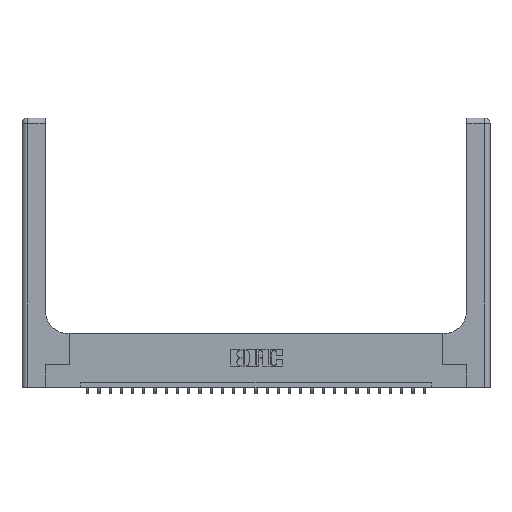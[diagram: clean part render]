
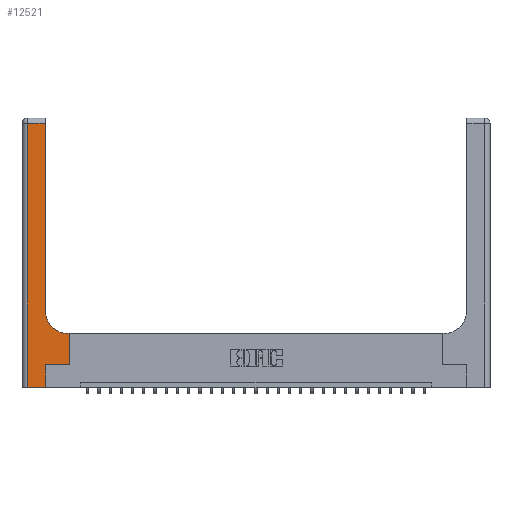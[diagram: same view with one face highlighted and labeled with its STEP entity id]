
A CAD part, top view. The second image highlights one B-rep face of the part: STEP entity #12521.
In plain terms, the highlighted planar face has unit normal (0, 0, 1).
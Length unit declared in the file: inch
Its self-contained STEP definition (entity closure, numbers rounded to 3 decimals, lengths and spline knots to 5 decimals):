
#50 = DIRECTION ( 'NONE',  ( 1., 0., 0. ) ) ;
#111 = CARTESIAN_POINT ( 'NONE',  ( 0.265, 0., 0.37 ) ) ;
#427 = VERTEX_POINT ( 'NONE', #14465 ) ;
#532 = ORIENTED_EDGE ( 'NONE', *, *, #23158, .T. ) ;
#588 = CARTESIAN_POINT ( 'NONE',  ( 0.528, 0.6, 0.37 ) ) ;
#691 = VECTOR ( 'NONE', #22587, 39.37008 ) ;
#862 = ORIENTED_EDGE ( 'NONE', *, *, #18617, .T. ) ;
#1159 = CARTESIAN_POINT ( 'NONE',  ( 0.528, 0.25, 0.37 ) ) ;
#1167 = ORIENTED_EDGE ( 'NONE', *, *, #24112, .T. ) ;
#1760 = EDGE_CURVE ( 'NONE', #3355, #6102, #11628, .T. ) ;
#1954 = ORIENTED_EDGE ( 'NONE', *, *, #11240, .T. ) ;
#2150 = DIRECTION ( 'NONE',  ( 0., 1., 0. ) ) ;
#2804 = AXIS2_PLACEMENT_3D ( 'NONE', #19322, #7292, #21332 ) ;
#3355 = VERTEX_POINT ( 'NONE', #23762 ) ;
#4939 = ORIENTED_EDGE ( 'NONE', *, *, #1760, .T. ) ;
#4972 = CARTESIAN_POINT ( 'NONE',  ( 0.06, 2.94, 0.37 ) ) ;
#5328 = EDGE_CURVE ( 'NONE', #8475, #16915, #11083, .T. ) ;
#5353 = DIRECTION ( 'NONE',  ( 0., 1., 0. ) ) ;
#5965 = CIRCLE ( 'NONE', #2804, 0.25 ) ;
#6033 = FACE_OUTER_BOUND ( 'NONE', #18383, .T. ) ;
#6042 = PLANE ( 'NONE',  #8187 ) ;
#6102 = VERTEX_POINT ( 'NONE', #4972 ) ;
#7292 = DIRECTION ( 'NONE',  ( 0., 0., -1. ) ) ;
#7917 = LINE ( 'NONE', #20095, #23245 ) ;
#8114 = DIRECTION ( 'NONE',  ( 0., 0., -1. ) ) ;
#8163 = LINE ( 'NONE', #12477, #17531 ) ;
#8187 = AXIS2_PLACEMENT_3D ( 'NONE', #24016, #8114, #22113 ) ;
#8475 = VERTEX_POINT ( 'NONE', #588 ) ;
#8661 = LINE ( 'NONE', #23739, #18674 ) ;
#9267 = LINE ( 'NONE', #111, #18015 ) ;
#9355 = EDGE_CURVE ( 'NONE', #427, #17977, #8661, .T. ) ;
#9898 = EDGE_CURVE ( 'NONE', #12443, #427, #9267, .T. ) ;
#10510 = DIRECTION ( 'NONE',  ( -1., 0., 0. ) ) ;
#10623 = CARTESIAN_POINT ( 'NONE',  ( 0.06, 3., 0.37 ) ) ;
#11083 = LINE ( 'NONE', #24469, #21079 ) ;
#11094 = VERTEX_POINT ( 'NONE', #13702 ) ;
#11240 = EDGE_CURVE ( 'NONE', #11094, #12443, #7917, .T. ) ;
#11435 = LINE ( 'NONE', #10623, #691 ) ;
#11628 = LINE ( 'NONE', #15218, #15021 ) ;
#11678 = ORIENTED_EDGE ( 'NONE', *, *, #9898, .T. ) ;
#12443 = VERTEX_POINT ( 'NONE', #23836 ) ;
#12477 = CARTESIAN_POINT ( 'NONE',  ( 0.528, 0.25, 0.37 ) ) ;
#12521 = ADVANCED_FACE ( 'NONE', ( #6033 ), #6042, .F. ) ;
#13414 = VECTOR ( 'NONE', #5353, 39.37008 ) ;
#13702 = CARTESIAN_POINT ( 'NONE',  ( 0.06, 0., 0.37 ) ) ;
#13934 = ORIENTED_EDGE ( 'NONE', *, *, #9355, .T. ) ;
#14465 = CARTESIAN_POINT ( 'NONE',  ( 0.265, 0.25, 0.37 ) ) ;
#15021 = VECTOR ( 'NONE', #21262, 39.37008 ) ;
#15218 = CARTESIAN_POINT ( 'NONE',  ( 0., 2.94, 0.37 ) ) ;
#15515 = CARTESIAN_POINT ( 'NONE',  ( 0.26, 0.85, 0.37 ) ) ;
#16285 = ORIENTED_EDGE ( 'NONE', *, *, #5328, .T. ) ;
#16915 = VERTEX_POINT ( 'NONE', #17501 ) ;
#17066 = ORIENTED_EDGE ( 'NONE', *, *, #21634, .T. ) ;
#17501 = CARTESIAN_POINT ( 'NONE',  ( 0.51, 0.6, 0.37 ) ) ;
#17531 = VECTOR ( 'NONE', #24419, 39.37008 ) ;
#17977 = VERTEX_POINT ( 'NONE', #1159 ) ;
#18015 = VECTOR ( 'NONE', #2150, 39.37008 ) ;
#18383 = EDGE_LOOP ( 'NONE', ( #862, #4939, #17066, #1954, #11678, #13934, #1167, #16285, #532 ) ) ;
#18617 = EDGE_CURVE ( 'NONE', #25526, #3355, #24050, .T. ) ;
#18674 = VECTOR ( 'NONE', #25737, 39.37008 ) ;
#19322 = CARTESIAN_POINT ( 'NONE',  ( 0.51, 0.85, 0.37 ) ) ;
#20095 = CARTESIAN_POINT ( 'NONE',  ( 0., 0., 0.37 ) ) ;
#21079 = VECTOR ( 'NONE', #10510, 39.37008 ) ;
#21262 = DIRECTION ( 'NONE',  ( -1., 0., 0. ) ) ;
#21332 = DIRECTION ( 'NONE',  ( 1., 0., 0. ) ) ;
#21634 = EDGE_CURVE ( 'NONE', #6102, #11094, #11435, .T. ) ;
#22113 = DIRECTION ( 'NONE',  ( -1., 0., 0. ) ) ;
#22587 = DIRECTION ( 'NONE',  ( 0., -1., 0. ) ) ;
#23158 = EDGE_CURVE ( 'NONE', #16915, #25526, #5965, .T. ) ;
#23245 = VECTOR ( 'NONE', #50, 39.37008 ) ;
#23739 = CARTESIAN_POINT ( 'NONE',  ( 0.265, 0.25, 0.37 ) ) ;
#23762 = CARTESIAN_POINT ( 'NONE',  ( 0.26, 2.94, 0.37 ) ) ;
#23836 = CARTESIAN_POINT ( 'NONE',  ( 0.265, 0., 0.37 ) ) ;
#24016 = CARTESIAN_POINT ( 'NONE',  ( 0., 3., 0.37 ) ) ;
#24050 = LINE ( 'NONE', #25420, #13414 ) ;
#24112 = EDGE_CURVE ( 'NONE', #17977, #8475, #8163, .T. ) ;
#24419 = DIRECTION ( 'NONE',  ( 0., 1., 0. ) ) ;
#24469 = CARTESIAN_POINT ( 'NONE',  ( 0.26, 0.6, 0.37 ) ) ;
#25420 = CARTESIAN_POINT ( 'NONE',  ( 0.26, 3., 0.37 ) ) ;
#25526 = VERTEX_POINT ( 'NONE', #15515 ) ;
#25737 = DIRECTION ( 'NONE',  ( 1., 0., 0. ) ) ;
